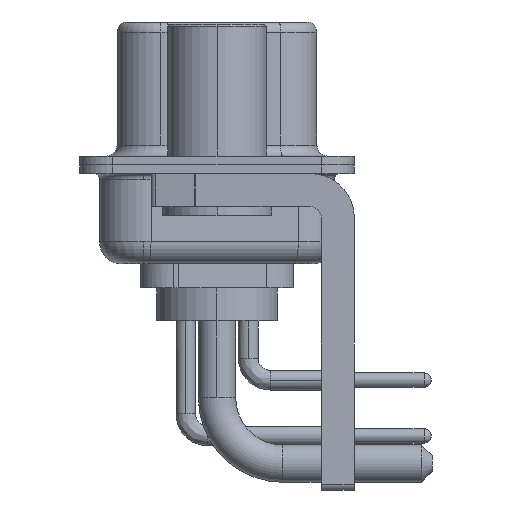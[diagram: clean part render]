
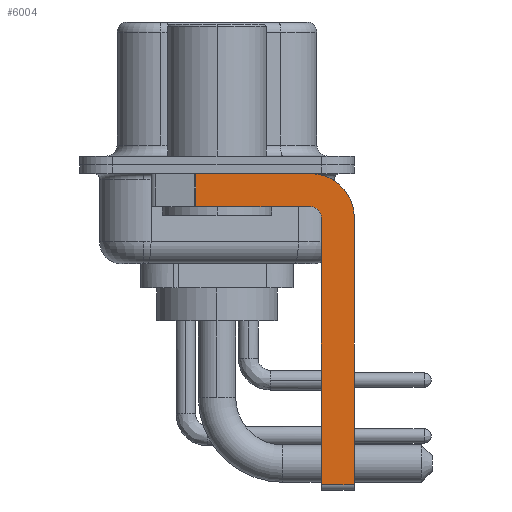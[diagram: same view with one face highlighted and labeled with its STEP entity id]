
A CAD part, left-side view. The second image highlights one B-rep face of the part: STEP entity #6004.
In plain terms, the highlighted planar face has unit normal (-1, 0, 0).
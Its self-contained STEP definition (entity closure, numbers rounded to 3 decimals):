
#252 = DIRECTION ( 'NONE',  ( 0., 0., 1. ) ) ;
#592 = CARTESIAN_POINT ( 'NONE',  ( -2.9, -4.25, -1.9 ) ) ;
#1113 = DIRECTION ( 'NONE',  ( 0., -1., 0. ) ) ;
#1462 = ORIENTED_EDGE ( 'NONE', *, *, #13839, .F. ) ;
#1577 = CARTESIAN_POINT ( 'NONE',  ( -2.9, 0.978, -1.9 ) ) ;
#1633 = CARTESIAN_POINT ( 'NONE',  ( -2.9, 0.978, -1.9 ) ) ;
#1636 = EDGE_CURVE ( 'NONE', #14180, #13162, #11949, .T. ) ;
#2228 = EDGE_CURVE ( 'NONE', #12893, #13142, #3244, .T. ) ;
#2600 = ORIENTED_EDGE ( 'NONE', *, *, #12578, .F. ) ;
#2644 = DIRECTION ( 'NONE',  ( 0., 1., 0. ) ) ;
#3244 = CIRCLE ( 'NONE', #24181, 2. ) ;
#3665 = DIRECTION ( 'NONE',  ( 0., 0., -1. ) ) ;
#3708 = CARTESIAN_POINT ( 'NONE',  ( -2.9, -4.25, -2.4 ) ) ;
#4014 = CARTESIAN_POINT ( 'NONE',  ( -2.9, -4.25, -2.4 ) ) ;
#4201 = CARTESIAN_POINT ( 'NONE',  ( -2.9, -6.25, -2.4 ) ) ;
#4564 = DIRECTION ( 'NONE',  ( 1., 0., 0. ) ) ;
#5177 = EDGE_LOOP ( 'NONE', ( #1462, #22625, #22099, #2600, #6715, #21147, #19224, #11726 ) ) ;
#6004 = ADVANCED_FACE ( 'NONE', ( #18497 ), #16720, .F. ) ;
#6715 = ORIENTED_EDGE ( 'NONE', *, *, #24232, .F. ) ;
#7857 = DIRECTION ( 'NONE',  ( 0., -1., 0. ) ) ;
#8028 = AXIS2_PLACEMENT_3D ( 'NONE', #18443, #26768, #252 ) ;
#8450 = CIRCLE ( 'NONE', #8028, 0.5 ) ;
#9018 = VERTEX_POINT ( 'NONE', #1633 ) ;
#9186 = CARTESIAN_POINT ( 'NONE',  ( -2.9, -4.75, -2.4 ) ) ;
#9453 = AXIS2_PLACEMENT_3D ( 'NONE', #4014, #4564, #21069 ) ;
#9501 = CARTESIAN_POINT ( 'NONE',  ( -2.9, -4.25, -14.55 ) ) ;
#10167 = VECTOR ( 'NONE', #12746, 1000. ) ;
#10265 = CARTESIAN_POINT ( 'NONE',  ( -2.9, 0.978, -0.4 ) ) ;
#10481 = VERTEX_POINT ( 'NONE', #16802 ) ;
#10960 = EDGE_CURVE ( 'NONE', #10481, #9018, #17549, .T. ) ;
#11382 = VECTOR ( 'NONE', #3665, 1000. ) ;
#11726 = ORIENTED_EDGE ( 'NONE', *, *, #2228, .F. ) ;
#11949 = LINE ( 'NONE', #9501, #25036 ) ;
#12053 = DIRECTION ( 'NONE',  ( 1., 0., 0. ) ) ;
#12578 = EDGE_CURVE ( 'NONE', #24844, #10481, #8450, .T. ) ;
#12640 = VECTOR ( 'NONE', #2644, 1000. ) ;
#12746 = DIRECTION ( 'NONE',  ( 0., 0., 1. ) ) ;
#12893 = VERTEX_POINT ( 'NONE', #22374 ) ;
#13142 = VERTEX_POINT ( 'NONE', #16492 ) ;
#13162 = VERTEX_POINT ( 'NONE', #18942 ) ;
#13839 = EDGE_CURVE ( 'NONE', #26334, #12893, #21754, .T. ) ;
#14180 = VERTEX_POINT ( 'NONE', #25275 ) ;
#14917 = CARTESIAN_POINT ( 'NONE',  ( -2.9, -4.75, -14.8 ) ) ;
#16408 = DIRECTION ( 'NONE',  ( 0., 0., -1. ) ) ;
#16492 = CARTESIAN_POINT ( 'NONE',  ( -2.9, -6.25, -2.4 ) ) ;
#16667 = VECTOR ( 'NONE', #1113, 1000. ) ;
#16720 = PLANE ( 'NONE',  #9453 ) ;
#16802 = CARTESIAN_POINT ( 'NONE',  ( -2.9, -4.25, -1.9 ) ) ;
#16984 = LINE ( 'NONE', #14917, #10167 ) ;
#17549 = LINE ( 'NONE', #592, #12640 ) ;
#18443 = CARTESIAN_POINT ( 'NONE',  ( -2.9, -4.25, -2.4 ) ) ;
#18497 = FACE_OUTER_BOUND ( 'NONE', #5177, .T. ) ;
#18588 = EDGE_CURVE ( 'NONE', #26334, #9018, #20300, .T. ) ;
#18942 = CARTESIAN_POINT ( 'NONE',  ( -2.9, -6.25, -14.55 ) ) ;
#19224 = ORIENTED_EDGE ( 'NONE', *, *, #21917, .F. ) ;
#20300 = LINE ( 'NONE', #1577, #20877 ) ;
#20877 = VECTOR ( 'NONE', #24668, 1000. ) ;
#21069 = DIRECTION ( 'NONE',  ( 0., 0., -1. ) ) ;
#21147 = ORIENTED_EDGE ( 'NONE', *, *, #1636, .T. ) ;
#21754 = LINE ( 'NONE', #23809, #16667 ) ;
#21917 = EDGE_CURVE ( 'NONE', #13142, #13162, #22908, .T. ) ;
#22099 = ORIENTED_EDGE ( 'NONE', *, *, #10960, .F. ) ;
#22374 = CARTESIAN_POINT ( 'NONE',  ( -2.9, -4.25, -0.4 ) ) ;
#22625 = ORIENTED_EDGE ( 'NONE', *, *, #18588, .T. ) ;
#22908 = LINE ( 'NONE', #4201, #11382 ) ;
#23809 = CARTESIAN_POINT ( 'NONE',  ( -2.9, 3., -0.4 ) ) ;
#24181 = AXIS2_PLACEMENT_3D ( 'NONE', #3708, #12053, #16408 ) ;
#24232 = EDGE_CURVE ( 'NONE', #14180, #24844, #16984, .T. ) ;
#24668 = DIRECTION ( 'NONE',  ( 0., 0., -1. ) ) ;
#24844 = VERTEX_POINT ( 'NONE', #9186 ) ;
#25036 = VECTOR ( 'NONE', #7857, 1000. ) ;
#25275 = CARTESIAN_POINT ( 'NONE',  ( -2.9, -4.75, -14.55 ) ) ;
#26334 = VERTEX_POINT ( 'NONE', #10265 ) ;
#26768 = DIRECTION ( 'NONE',  ( -1., 0., 0. ) ) ;
